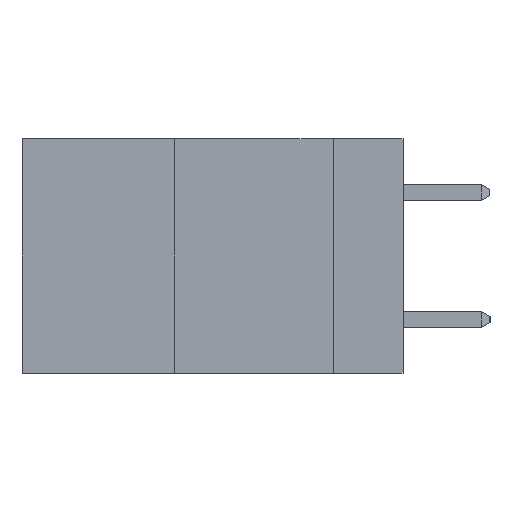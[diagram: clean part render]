
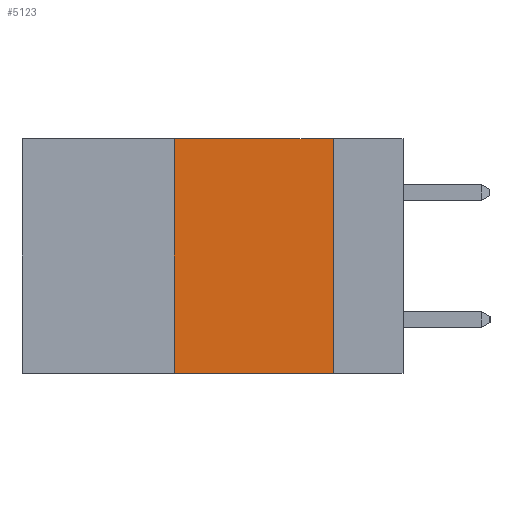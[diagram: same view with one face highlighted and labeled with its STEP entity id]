
A CAD part, left-side view. The second image highlights one B-rep face of the part: STEP entity #5123.
In plain terms, the highlighted planar face has unit normal (-1, 0, 0).
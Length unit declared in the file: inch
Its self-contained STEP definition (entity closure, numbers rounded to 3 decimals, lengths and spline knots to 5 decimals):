
#544 = LINE ( 'NONE', #8825, #7925 ) ;
#655 = VECTOR ( 'NONE', #10714, 39.37008 ) ;
#1421 = ORIENTED_EDGE ( 'NONE', *, *, #2786, .F. ) ;
#1936 = ORIENTED_EDGE ( 'NONE', *, *, #3014, .F. ) ;
#2410 = DIRECTION ( 'NONE',  ( 0., 0., -1. ) ) ;
#2786 = EDGE_CURVE ( 'NONE', #6447, #9907, #11669, .T. ) ;
#3014 = EDGE_CURVE ( 'NONE', #9907, #3060, #8531, .T. ) ;
#3060 = VERTEX_POINT ( 'NONE', #8529 ) ;
#3439 = CARTESIAN_POINT ( 'NONE',  ( 0., 0.36, -0.37 ) ) ;
#3558 = ORIENTED_EDGE ( 'NONE', *, *, #7495, .T. ) ;
#3644 = DIRECTION ( 'NONE',  ( 0., 0., -1. ) ) ;
#5123 = ADVANCED_FACE ( 'NONE', ( #7671 ), #11949, .F. ) ;
#5659 = CARTESIAN_POINT ( 'NONE',  ( 0., 0.6, 0. ) ) ;
#5735 = VECTOR ( 'NONE', #2410, 39.37008 ) ;
#6447 = VERTEX_POINT ( 'NONE', #8277 ) ;
#7081 = CARTESIAN_POINT ( 'NONE',  ( 0., 0.11, 0. ) ) ;
#7331 = VERTEX_POINT ( 'NONE', #3439 ) ;
#7495 = EDGE_CURVE ( 'NONE', #7331, #3060, #544, .T. ) ;
#7527 = CARTESIAN_POINT ( 'NONE',  ( 0., 0.6, 0. ) ) ;
#7671 = FACE_OUTER_BOUND ( 'NONE', #12017, .T. ) ;
#7768 = DIRECTION ( 'NONE',  ( 1., 0., 0. ) ) ;
#7925 = VECTOR ( 'NONE', #9901, 39.37008 ) ;
#8127 = ORIENTED_EDGE ( 'NONE', *, *, #9819, .F. ) ;
#8277 = CARTESIAN_POINT ( 'NONE',  ( 0., 0.36, 0. ) ) ;
#8529 = CARTESIAN_POINT ( 'NONE',  ( 0., 0.11, -0.37 ) ) ;
#8531 = LINE ( 'NONE', #8582, #5735 ) ;
#8582 = CARTESIAN_POINT ( 'NONE',  ( 0., 0.11, 0. ) ) ;
#8825 = CARTESIAN_POINT ( 'NONE',  ( 0., 0.6, -0.37 ) ) ;
#9819 = EDGE_CURVE ( 'NONE', #7331, #6447, #13435, .T. ) ;
#9901 = DIRECTION ( 'NONE',  ( 0., -1., 0. ) ) ;
#9907 = VERTEX_POINT ( 'NONE', #7081 ) ;
#10314 = VECTOR ( 'NONE', #10857, 39.37008 ) ;
#10714 = DIRECTION ( 'NONE',  ( 0., -1., 0. ) ) ;
#10857 = DIRECTION ( 'NONE',  ( 0., 0., 1. ) ) ;
#10994 = AXIS2_PLACEMENT_3D ( 'NONE', #5659, #7768, #3644 ) ;
#11669 = LINE ( 'NONE', #7527, #655 ) ;
#11772 = CARTESIAN_POINT ( 'NONE',  ( 0., 0.36, 0. ) ) ;
#11949 = PLANE ( 'NONE',  #10994 ) ;
#12017 = EDGE_LOOP ( 'NONE', ( #1936, #1421, #8127, #3558 ) ) ;
#13435 = LINE ( 'NONE', #11772, #10314 ) ;
